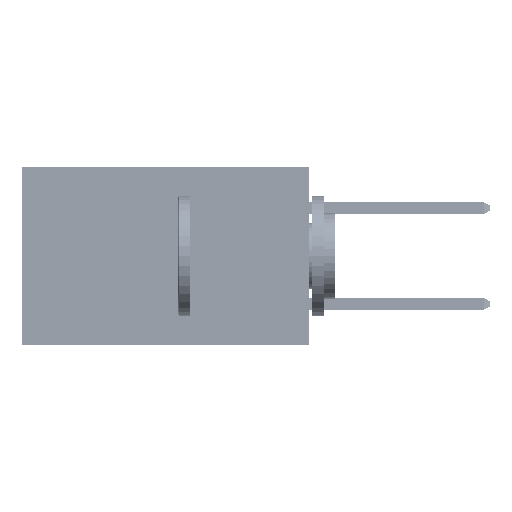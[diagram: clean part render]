
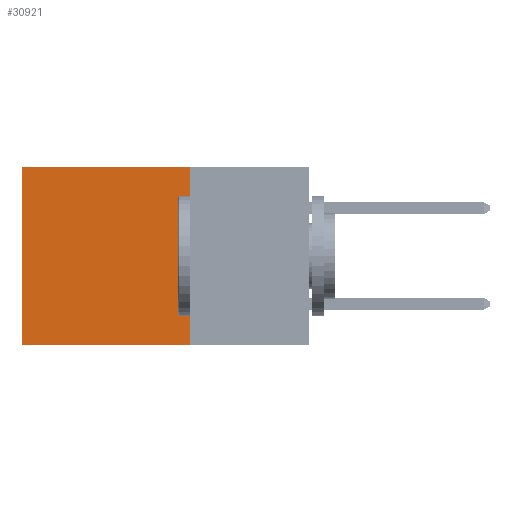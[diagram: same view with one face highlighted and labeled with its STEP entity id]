
A CAD part, left-side view. The second image highlights one B-rep face of the part: STEP entity #30921.
In plain terms, the highlighted planar face has unit normal (-1, 0, 0).
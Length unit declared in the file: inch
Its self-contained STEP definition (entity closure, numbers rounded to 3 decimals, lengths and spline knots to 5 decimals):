
#951 = VERTEX_POINT ( 'NONE', #16206 ) ;
#1669 = VECTOR ( 'NONE', #21747, 39.37008 ) ;
#2730 = ORIENTED_EDGE ( 'NONE', *, *, #15971, .F. ) ;
#2871 = AXIS2_PLACEMENT_3D ( 'NONE', #45809, #49870, #25422 ) ;
#3440 = VERTEX_POINT ( 'NONE', #51351 ) ;
#4351 = CARTESIAN_POINT ( 'NONE',  ( 0.2875, 0.25, 0. ) ) ;
#6588 = CARTESIAN_POINT ( 'NONE',  ( 0.2875, 0.25, 0. ) ) ;
#8275 = ORIENTED_EDGE ( 'NONE', *, *, #44675, .F. ) ;
#8737 = PLANE ( 'NONE',  #2871 ) ;
#9511 = LINE ( 'NONE', #53137, #39853 ) ;
#12385 = EDGE_LOOP ( 'NONE', ( #32437, #2730, #8275, #41535 ) ) ;
#12451 = DIRECTION ( 'NONE',  ( 0., 1., 0. ) ) ;
#15574 = VERTEX_POINT ( 'NONE', #6588 ) ;
#15971 = EDGE_CURVE ( 'NONE', #951, #3440, #34675, .T. ) ;
#16206 = CARTESIAN_POINT ( 'NONE',  ( 0.2875, 0.25, -0.37 ) ) ;
#17628 = CARTESIAN_POINT ( 'NONE',  ( 0.2875, 0.25, -0.37 ) ) ;
#17703 = LINE ( 'NONE', #46091, #38320 ) ;
#21747 = DIRECTION ( 'NONE',  ( 0., 1., 0. ) ) ;
#24621 = DIRECTION ( 'NONE',  ( 0., 0., -1. ) ) ;
#25422 = DIRECTION ( 'NONE',  ( 0., 0., -1. ) ) ;
#27060 = VERTEX_POINT ( 'NONE', #49631 ) ;
#30921 = ADVANCED_FACE ( 'NONE', ( #51744 ), #8737, .F. ) ;
#31548 = VECTOR ( 'NONE', #12451, 39.37008 ) ;
#32437 = ORIENTED_EDGE ( 'NONE', *, *, #41840, .T. ) ;
#34675 = LINE ( 'NONE', #17628, #1669 ) ;
#38320 = VECTOR ( 'NONE', #50152, 39.37008 ) ;
#39853 = VECTOR ( 'NONE', #24621, 39.37008 ) ;
#41535 = ORIENTED_EDGE ( 'NONE', *, *, #50064, .T. ) ;
#41840 = EDGE_CURVE ( 'NONE', #27060, #3440, #17703, .T. ) ;
#44675 = EDGE_CURVE ( 'NONE', #15574, #951, #9511, .T. ) ;
#45809 = CARTESIAN_POINT ( 'NONE',  ( 0.2875, 0.25, 0. ) ) ;
#46091 = CARTESIAN_POINT ( 'NONE',  ( 0.2875, 0.6, 0. ) ) ;
#49631 = CARTESIAN_POINT ( 'NONE',  ( 0.2875, 0.6, 0. ) ) ;
#49870 = DIRECTION ( 'NONE',  ( 1., 0., 0. ) ) ;
#50064 = EDGE_CURVE ( 'NONE', #15574, #27060, #51830, .T. ) ;
#50152 = DIRECTION ( 'NONE',  ( 0., 0., -1. ) ) ;
#51351 = CARTESIAN_POINT ( 'NONE',  ( 0.2875, 0.6, -0.37 ) ) ;
#51744 = FACE_OUTER_BOUND ( 'NONE', #12385, .T. ) ;
#51830 = LINE ( 'NONE', #4351, #31548 ) ;
#53137 = CARTESIAN_POINT ( 'NONE',  ( 0.2875, 0.25, 0. ) ) ;
